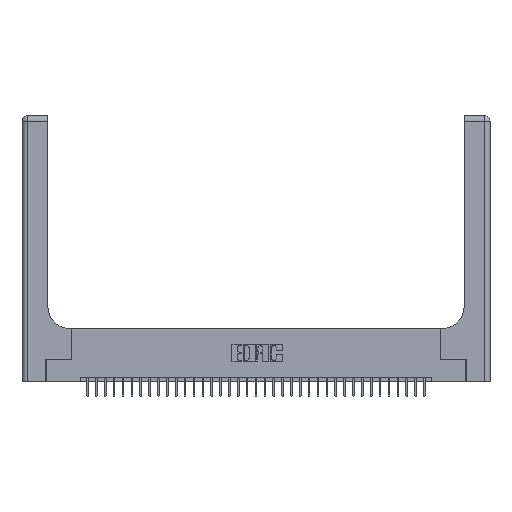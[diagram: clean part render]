
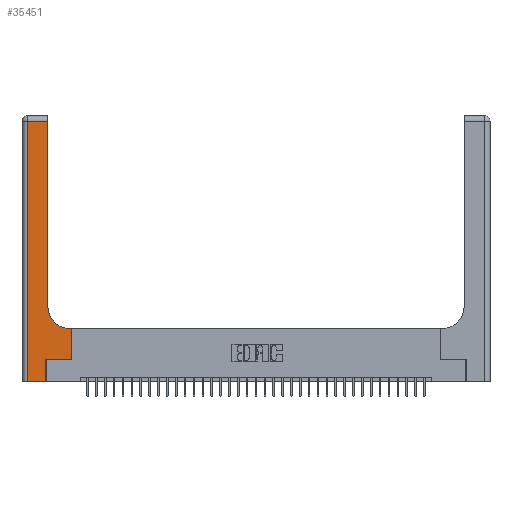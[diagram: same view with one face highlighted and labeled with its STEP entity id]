
A CAD part, top view. The second image highlights one B-rep face of the part: STEP entity #35451.
In plain terms, the highlighted planar face has unit normal (0, 0, 1).
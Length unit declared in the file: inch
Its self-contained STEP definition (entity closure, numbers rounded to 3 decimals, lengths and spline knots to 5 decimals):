
#240 = EDGE_CURVE ( 'NONE', #19934, #25792, #29441, .T. ) ;
#1570 = CARTESIAN_POINT ( 'NONE',  ( 0.269, 0.25, 0.37 ) ) ;
#1682 = CARTESIAN_POINT ( 'NONE',  ( 0., 0., 0.37 ) ) ;
#2566 = DIRECTION ( 'NONE',  ( 0., 0., -1. ) ) ;
#3214 = VERTEX_POINT ( 'NONE', #34743 ) ;
#3774 = EDGE_CURVE ( 'NONE', #25792, #28906, #22949, .T. ) ;
#4476 = CARTESIAN_POINT ( 'NONE',  ( 0.269, 0.25, 0.37 ) ) ;
#4676 = VERTEX_POINT ( 'NONE', #10851 ) ;
#4829 = CARTESIAN_POINT ( 'NONE',  ( 0.5585, 0.25, 0.37 ) ) ;
#7208 = ORIENTED_EDGE ( 'NONE', *, *, #22426, .T. ) ;
#7367 = LINE ( 'NONE', #32768, #27868 ) ;
#7456 = CARTESIAN_POINT ( 'NONE',  ( 0., 3., 0.37 ) ) ;
#7611 = LINE ( 'NONE', #25436, #27246 ) ;
#7670 = DIRECTION ( 'NONE',  ( 0., 1., 0. ) ) ;
#8549 = ORIENTED_EDGE ( 'NONE', *, *, #11315, .T. ) ;
#9433 = VECTOR ( 'NONE', #25529, 39.37008 ) ;
#10291 = PLANE ( 'NONE',  #27794 ) ;
#10851 = CARTESIAN_POINT ( 'NONE',  ( 0.5415, 0.6, 0.37 ) ) ;
#11226 = DIRECTION ( 'NONE',  ( 0., 1., 0. ) ) ;
#11315 = EDGE_CURVE ( 'NONE', #23919, #18992, #7367, .T. ) ;
#11841 = VERTEX_POINT ( 'NONE', #32431 ) ;
#12292 = CIRCLE ( 'NONE', #19624, 0.25 ) ;
#13118 = DIRECTION ( 'NONE',  ( -1., 0., 0. ) ) ;
#16437 = EDGE_CURVE ( 'NONE', #3214, #4676, #16860, .T. ) ;
#16860 = LINE ( 'NONE', #33717, #9433 ) ;
#17768 = CARTESIAN_POINT ( 'NONE',  ( 0.269, 0., 0.37 ) ) ;
#18269 = VECTOR ( 'NONE', #21354, 39.37008 ) ;
#18992 = VERTEX_POINT ( 'NONE', #25718 ) ;
#19431 = CARTESIAN_POINT ( 'NONE',  ( 0.5415, 0.85, 0.37 ) ) ;
#19624 = AXIS2_PLACEMENT_3D ( 'NONE', #19431, #2566, #22202 ) ;
#19934 = VERTEX_POINT ( 'NONE', #24416 ) ;
#20191 = CARTESIAN_POINT ( 'NONE',  ( 0.2915, 2.94, 0.37 ) ) ;
#20444 = ORIENTED_EDGE ( 'NONE', *, *, #32985, .T. ) ;
#21274 = ORIENTED_EDGE ( 'NONE', *, *, #22234, .T. ) ;
#21354 = DIRECTION ( 'NONE',  ( 1., 0., 0. ) ) ;
#21677 = DIRECTION ( 'NONE',  ( 0., -1., 0. ) ) ;
#22059 = VECTOR ( 'NONE', #23929, 39.37008 ) ;
#22066 = VECTOR ( 'NONE', #28915, 39.37008 ) ;
#22173 = EDGE_CURVE ( 'NONE', #18992, #19934, #32970, .T. ) ;
#22202 = DIRECTION ( 'NONE',  ( 1., 0., 0. ) ) ;
#22234 = EDGE_CURVE ( 'NONE', #28906, #3214, #23053, .T. ) ;
#22426 = EDGE_CURVE ( 'NONE', #11841, #28984, #30810, .T. ) ;
#22949 = LINE ( 'NONE', #4476, #22059 ) ;
#23053 = LINE ( 'NONE', #4829, #29536 ) ;
#23464 = VECTOR ( 'NONE', #11226, 39.37008 ) ;
#23854 = ORIENTED_EDGE ( 'NONE', *, *, #22173, .T. ) ;
#23919 = VERTEX_POINT ( 'NONE', #30202 ) ;
#23929 = DIRECTION ( 'NONE',  ( 1., 0., 0. ) ) ;
#24416 = CARTESIAN_POINT ( 'NONE',  ( 0.269, 0., 0.37 ) ) ;
#25109 = CARTESIAN_POINT ( 'NONE',  ( 0.2915, 3., 0.37 ) ) ;
#25431 = CARTESIAN_POINT ( 'NONE',  ( 0.5585, 0.25, 0.37 ) ) ;
#25436 = CARTESIAN_POINT ( 'NONE',  ( 0., 2.94, 0.37 ) ) ;
#25529 = DIRECTION ( 'NONE',  ( -1., 0., 0. ) ) ;
#25684 = DIRECTION ( 'NONE',  ( -1., 0., 0. ) ) ;
#25718 = CARTESIAN_POINT ( 'NONE',  ( 0.06, 0., 0.37 ) ) ;
#25780 = FACE_OUTER_BOUND ( 'NONE', #29396, .T. ) ;
#25792 = VERTEX_POINT ( 'NONE', #1570 ) ;
#26060 = ORIENTED_EDGE ( 'NONE', *, *, #3774, .T. ) ;
#27246 = VECTOR ( 'NONE', #25684, 39.37008 ) ;
#27372 = ORIENTED_EDGE ( 'NONE', *, *, #16437, .T. ) ;
#27794 = AXIS2_PLACEMENT_3D ( 'NONE', #7456, #29736, #13118 ) ;
#27868 = VECTOR ( 'NONE', #21677, 39.37008 ) ;
#28906 = VERTEX_POINT ( 'NONE', #25431 ) ;
#28915 = DIRECTION ( 'NONE',  ( 0., 1., 0. ) ) ;
#28984 = VERTEX_POINT ( 'NONE', #20191 ) ;
#29396 = EDGE_LOOP ( 'NONE', ( #7208, #31175, #8549, #23854, #33803, #26060, #21274, #27372, #20444 ) ) ;
#29441 = LINE ( 'NONE', #17768, #22066 ) ;
#29536 = VECTOR ( 'NONE', #7670, 39.37008 ) ;
#29736 = DIRECTION ( 'NONE',  ( 0., 0., -1. ) ) ;
#29891 = EDGE_CURVE ( 'NONE', #28984, #23919, #7611, .T. ) ;
#30202 = CARTESIAN_POINT ( 'NONE',  ( 0.06, 2.94, 0.37 ) ) ;
#30810 = LINE ( 'NONE', #25109, #23464 ) ;
#31175 = ORIENTED_EDGE ( 'NONE', *, *, #29891, .T. ) ;
#32431 = CARTESIAN_POINT ( 'NONE',  ( 0.2915, 0.85, 0.37 ) ) ;
#32768 = CARTESIAN_POINT ( 'NONE',  ( 0.06, 3., 0.37 ) ) ;
#32970 = LINE ( 'NONE', #1682, #18269 ) ;
#32985 = EDGE_CURVE ( 'NONE', #4676, #11841, #12292, .T. ) ;
#33717 = CARTESIAN_POINT ( 'NONE',  ( 0.2915, 0.6, 0.37 ) ) ;
#33803 = ORIENTED_EDGE ( 'NONE', *, *, #240, .T. ) ;
#34743 = CARTESIAN_POINT ( 'NONE',  ( 0.5585, 0.6, 0.37 ) ) ;
#35451 = ADVANCED_FACE ( 'NONE', ( #25780 ), #10291, .F. ) ;
